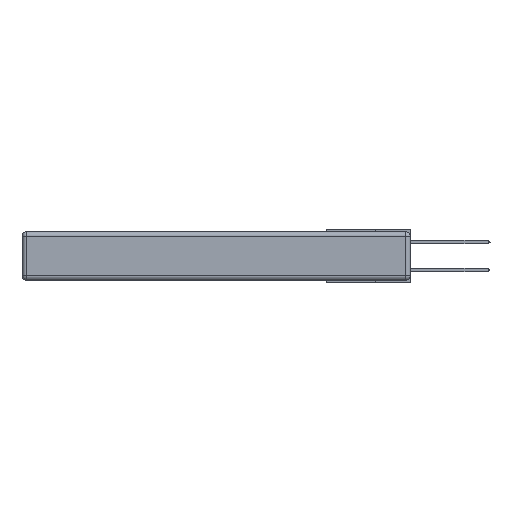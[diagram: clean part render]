
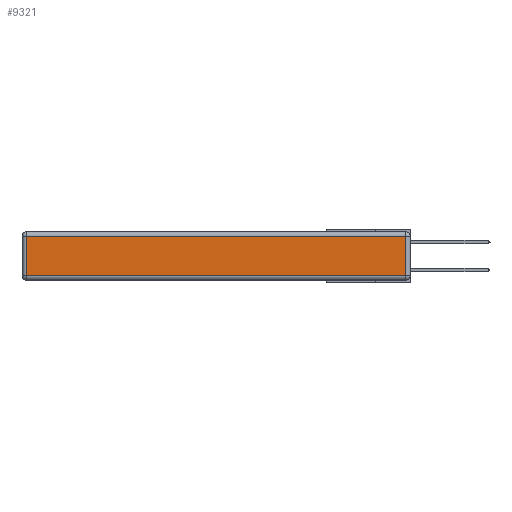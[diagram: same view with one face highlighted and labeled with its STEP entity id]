
A CAD part, left-side view. The second image highlights one B-rep face of the part: STEP entity #9321.
In plain terms, the highlighted planar face has unit normal (-1, 0, 0).
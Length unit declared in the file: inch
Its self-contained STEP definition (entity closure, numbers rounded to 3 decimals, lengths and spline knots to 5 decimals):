
#227 = VERTEX_POINT ( 'NONE', #14854 ) ;
#1042 = EDGE_CURVE ( 'NONE', #12546, #17566, #13276, .T. ) ;
#2763 = CARTESIAN_POINT ( 'NONE',  ( 0., 0.03, -0.343 ) ) ;
#3191 = LINE ( 'NONE', #7165, #11630 ) ;
#4019 = CARTESIAN_POINT ( 'NONE',  ( 0., 2.72, -0.313 ) ) ;
#4720 = VECTOR ( 'NONE', #15141, 39.37008 ) ;
#5629 = EDGE_LOOP ( 'NONE', ( #11283, #17847, #18507, #15249 ) ) ;
#6938 = EDGE_CURVE ( 'NONE', #227, #12546, #9199, .T. ) ;
#7165 = CARTESIAN_POINT ( 'NONE',  ( 0., 2.75, -0.03 ) ) ;
#8294 = FACE_OUTER_BOUND ( 'NONE', #5629, .T. ) ;
#8775 = CARTESIAN_POINT ( 'NONE',  ( 0., 0., -0.343 ) ) ;
#8832 = EDGE_CURVE ( 'NONE', #17566, #19665, #14336, .T. ) ;
#9199 = LINE ( 'NONE', #17120, #4720 ) ;
#9321 = ADVANCED_FACE ( 'NONE', ( #8294 ), #10510, .T. ) ;
#9978 = CARTESIAN_POINT ( 'NONE',  ( 0., 0.03, -0.03 ) ) ;
#10479 = DIRECTION ( 'NONE',  ( 0., 0., 1. ) ) ;
#10510 = PLANE ( 'NONE',  #18596 ) ;
#11283 = ORIENTED_EDGE ( 'NONE', *, *, #1042, .T. ) ;
#11630 = VECTOR ( 'NONE', #15599, 39.37008 ) ;
#12209 = CARTESIAN_POINT ( 'NONE',  ( 0., 0.03, -0.313 ) ) ;
#12546 = VERTEX_POINT ( 'NONE', #4019 ) ;
#13276 = LINE ( 'NONE', #21319, #16937 ) ;
#14336 = LINE ( 'NONE', #2763, #15908 ) ;
#14618 = DIRECTION ( 'NONE',  ( 0., -1., 0. ) ) ;
#14854 = CARTESIAN_POINT ( 'NONE',  ( 0., 2.72, -0.03 ) ) ;
#15141 = DIRECTION ( 'NONE',  ( 0., 0., -1. ) ) ;
#15249 = ORIENTED_EDGE ( 'NONE', *, *, #6938, .T. ) ;
#15599 = DIRECTION ( 'NONE',  ( 0., 1., 0. ) ) ;
#15649 = DIRECTION ( 'NONE',  ( -1., 0., 0. ) ) ;
#15908 = VECTOR ( 'NONE', #18107, 39.37008 ) ;
#16906 = EDGE_CURVE ( 'NONE', #19665, #227, #3191, .T. ) ;
#16937 = VECTOR ( 'NONE', #14618, 39.37008 ) ;
#17120 = CARTESIAN_POINT ( 'NONE',  ( 0., 2.72, -0.343 ) ) ;
#17566 = VERTEX_POINT ( 'NONE', #12209 ) ;
#17847 = ORIENTED_EDGE ( 'NONE', *, *, #8832, .T. ) ;
#18107 = DIRECTION ( 'NONE',  ( 0., 0., 1. ) ) ;
#18507 = ORIENTED_EDGE ( 'NONE', *, *, #16906, .T. ) ;
#18596 = AXIS2_PLACEMENT_3D ( 'NONE', #8775, #15649, #10479 ) ;
#19665 = VERTEX_POINT ( 'NONE', #9978 ) ;
#21319 = CARTESIAN_POINT ( 'NONE',  ( 0., 0., -0.313 ) ) ;
